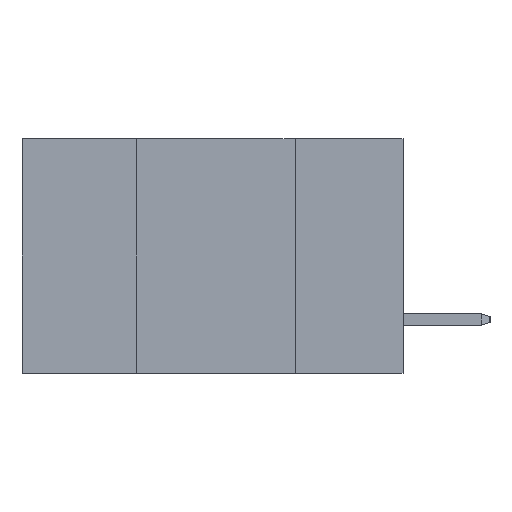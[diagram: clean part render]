
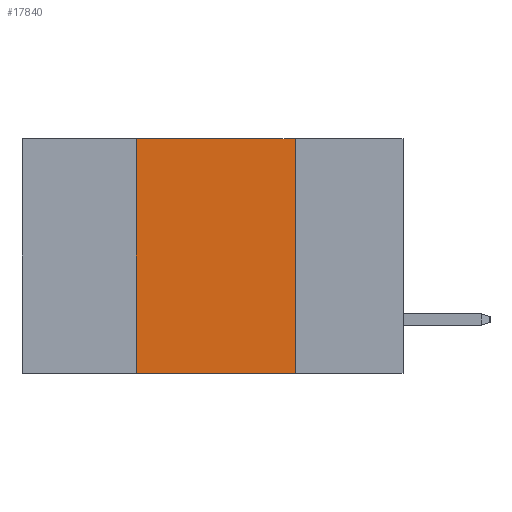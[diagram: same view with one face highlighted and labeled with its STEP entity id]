
A CAD part, left-side view. The second image highlights one B-rep face of the part: STEP entity #17840.
In plain terms, the highlighted planar face has unit normal (-1, 0, 0).
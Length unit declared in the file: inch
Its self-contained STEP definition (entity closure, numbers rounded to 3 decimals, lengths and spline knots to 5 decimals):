
#257 = LINE ( 'NONE', #1507, #3513 ) ;
#1507 = CARTESIAN_POINT ( 'NONE',  ( 0., 0.17, 0. ) ) ;
#2329 = VERTEX_POINT ( 'NONE', #15474 ) ;
#2380 = PLANE ( 'NONE',  #3541 ) ;
#3513 = VECTOR ( 'NONE', #7410, 39.37008 ) ;
#3541 = AXIS2_PLACEMENT_3D ( 'NONE', #15523, #11241, #8285 ) ;
#4972 = DIRECTION ( 'NONE',  ( 0., -1., 0. ) ) ;
#6022 = EDGE_CURVE ( 'NONE', #12785, #13269, #8127, .T. ) ;
#6097 = DIRECTION ( 'NONE',  ( 0., -1., 0. ) ) ;
#7410 = DIRECTION ( 'NONE',  ( 0., 0., -1. ) ) ;
#7423 = CARTESIAN_POINT ( 'NONE',  ( 0., 0.6, -0.37 ) ) ;
#7434 = VECTOR ( 'NONE', #4972, 39.37008 ) ;
#7511 = DIRECTION ( 'NONE',  ( 0., 0., 1. ) ) ;
#7555 = EDGE_CURVE ( 'NONE', #2329, #12785, #13116, .T. ) ;
#8127 = LINE ( 'NONE', #13920, #7434 ) ;
#8285 = DIRECTION ( 'NONE',  ( 0., 0., -1. ) ) ;
#8460 = VERTEX_POINT ( 'NONE', #9065 ) ;
#8787 = ORIENTED_EDGE ( 'NONE', *, *, #7555, .F. ) ;
#9065 = CARTESIAN_POINT ( 'NONE',  ( 0., 0.17, -0.37 ) ) ;
#9745 = ORIENTED_EDGE ( 'NONE', *, *, #6022, .F. ) ;
#10462 = LINE ( 'NONE', #7423, #11351 ) ;
#10588 = CARTESIAN_POINT ( 'NONE',  ( 0., 0.17, 0. ) ) ;
#11146 = FACE_OUTER_BOUND ( 'NONE', #12026, .T. ) ;
#11241 = DIRECTION ( 'NONE',  ( 1., 0., 0. ) ) ;
#11351 = VECTOR ( 'NONE', #6097, 39.37008 ) ;
#11434 = VECTOR ( 'NONE', #7511, 39.37008 ) ;
#12026 = EDGE_LOOP ( 'NONE', ( #15295, #9745, #8787, #12452 ) ) ;
#12274 = EDGE_CURVE ( 'NONE', #2329, #8460, #10462, .T. ) ;
#12452 = ORIENTED_EDGE ( 'NONE', *, *, #12274, .T. ) ;
#12785 = VERTEX_POINT ( 'NONE', #16414 ) ;
#13116 = LINE ( 'NONE', #17617, #11434 ) ;
#13269 = VERTEX_POINT ( 'NONE', #10588 ) ;
#13920 = CARTESIAN_POINT ( 'NONE',  ( 0., 0.6, 0. ) ) ;
#14984 = EDGE_CURVE ( 'NONE', #13269, #8460, #257, .T. ) ;
#15295 = ORIENTED_EDGE ( 'NONE', *, *, #14984, .F. ) ;
#15474 = CARTESIAN_POINT ( 'NONE',  ( 0., 0.42, -0.37 ) ) ;
#15523 = CARTESIAN_POINT ( 'NONE',  ( 0., 0.6, 0. ) ) ;
#16414 = CARTESIAN_POINT ( 'NONE',  ( 0., 0.42, 0. ) ) ;
#17617 = CARTESIAN_POINT ( 'NONE',  ( 0., 0.42, 0. ) ) ;
#17840 = ADVANCED_FACE ( 'NONE', ( #11146 ), #2380, .F. ) ;
